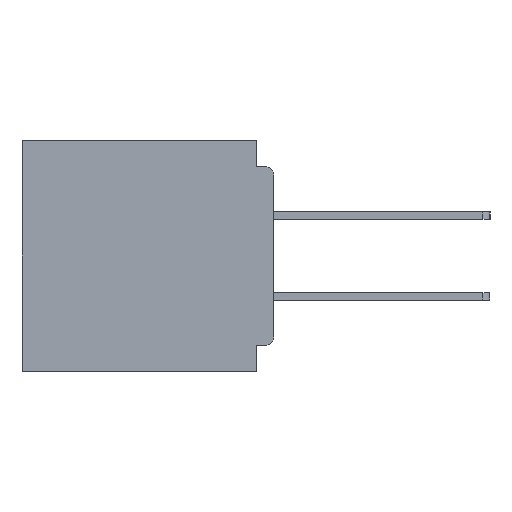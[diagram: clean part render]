
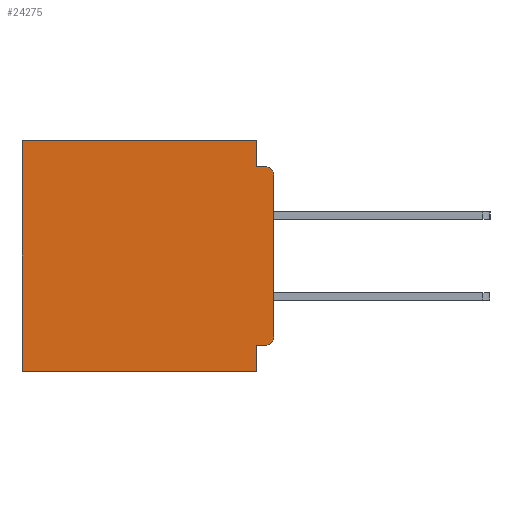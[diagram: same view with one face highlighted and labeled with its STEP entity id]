
A CAD part, left-side view. The second image highlights one B-rep face of the part: STEP entity #24275.
In plain terms, the highlighted planar face has unit normal (-1, 0, 0).
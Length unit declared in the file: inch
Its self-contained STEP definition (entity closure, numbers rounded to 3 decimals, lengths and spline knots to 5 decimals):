
#1259 = ORIENTED_EDGE ( 'NONE', *, *, #41364, .T. ) ;
#1896 = DIRECTION ( 'NONE',  ( 0., 0., -1. ) ) ;
#2210 = VECTOR ( 'NONE', #35630, 39.37008 ) ;
#3165 = CARTESIAN_POINT ( 'NONE',  ( 0.3, 0.015, -0.355 ) ) ;
#3655 = VERTEX_POINT ( 'NONE', #24168 ) ;
#3682 = AXIS2_PLACEMENT_3D ( 'NONE', #24047, #39330, #16484 ) ;
#4925 = CIRCLE ( 'NONE', #34473, 0.015 ) ;
#5330 = VERTEX_POINT ( 'NONE', #31087 ) ;
#6801 = EDGE_CURVE ( 'NONE', #7908, #34085, #31886, .T. ) ;
#6877 = LINE ( 'NONE', #7800, #17104 ) ;
#7800 = CARTESIAN_POINT ( 'NONE',  ( 0.3, 0., -0.355 ) ) ;
#7908 = VERTEX_POINT ( 'NONE', #9162 ) ;
#8068 = CARTESIAN_POINT ( 'NONE',  ( 0.3, 0., -0.4 ) ) ;
#8554 = ORIENTED_EDGE ( 'NONE', *, *, #32010, .F. ) ;
#9162 = CARTESIAN_POINT ( 'NONE',  ( 0.3, 0., -0.06 ) ) ;
#9656 = ORIENTED_EDGE ( 'NONE', *, *, #16237, .T. ) ;
#10289 = LINE ( 'NONE', #47189, #38359 ) ;
#10371 = CARTESIAN_POINT ( 'NONE',  ( 0.3, 0.015, -0.06 ) ) ;
#11651 = ORIENTED_EDGE ( 'NONE', *, *, #28597, .F. ) ;
#11797 = CARTESIAN_POINT ( 'NONE',  ( 0.3, 0., 0. ) ) ;
#12726 = CARTESIAN_POINT ( 'NONE',  ( 0.3, 0.437, -0.4 ) ) ;
#12987 = VECTOR ( 'NONE', #1896, 39.37008 ) ;
#13137 = EDGE_CURVE ( 'NONE', #5330, #17676, #21527, .T. ) ;
#14211 = DIRECTION ( 'NONE',  ( 0., 0., -1. ) ) ;
#16237 = EDGE_CURVE ( 'NONE', #43691, #34085, #44490, .T. ) ;
#16484 = DIRECTION ( 'NONE',  ( 0., 0., -1. ) ) ;
#17104 = VECTOR ( 'NONE', #34557, 39.37008 ) ;
#17636 = VERTEX_POINT ( 'NONE', #40933 ) ;
#17676 = VERTEX_POINT ( 'NONE', #19106 ) ;
#19106 = CARTESIAN_POINT ( 'NONE',  ( 0.3, 0.031, -0.4 ) ) ;
#20347 = VECTOR ( 'NONE', #34701, 39.37008 ) ;
#20806 = ORIENTED_EDGE ( 'NONE', *, *, #13137, .F. ) ;
#21331 = CARTESIAN_POINT ( 'NONE',  ( 0.3, 0., -0.34 ) ) ;
#21527 = LINE ( 'NONE', #24442, #41775 ) ;
#21607 = CARTESIAN_POINT ( 'NONE',  ( 0.3, 0.015, -0.34 ) ) ;
#24047 = CARTESIAN_POINT ( 'NONE',  ( 0.3, 0., -0.4 ) ) ;
#24168 = CARTESIAN_POINT ( 'NONE',  ( 0.3, 0.015, -0.045 ) ) ;
#24275 = ADVANCED_FACE ( 'NONE', ( #33967 ), #35515, .F. ) ;
#24442 = CARTESIAN_POINT ( 'NONE',  ( 0.3, 0.031, -0.4 ) ) ;
#25485 = DIRECTION ( 'NONE',  ( 0., 0., -1. ) ) ;
#25887 = EDGE_LOOP ( 'NONE', ( #32181, #32257, #46702, #11651, #42048, #1259, #27931, #20806, #8554, #9656 ) ) ;
#26176 = VECTOR ( 'NONE', #48220, 39.37008 ) ;
#27360 = LINE ( 'NONE', #44401, #26176 ) ;
#27374 = DIRECTION ( 'NONE',  ( 0., 0., -1. ) ) ;
#27720 = VERTEX_POINT ( 'NONE', #46425 ) ;
#27931 = ORIENTED_EDGE ( 'NONE', *, *, #38130, .F. ) ;
#28282 = DIRECTION ( 'NONE',  ( 0., 1., 0. ) ) ;
#28597 = EDGE_CURVE ( 'NONE', #27720, #44412, #33316, .T. ) ;
#29813 = EDGE_CURVE ( 'NONE', #44412, #3655, #27360, .T. ) ;
#30501 = LINE ( 'NONE', #11797, #20347 ) ;
#30678 = VERTEX_POINT ( 'NONE', #48464 ) ;
#31087 = CARTESIAN_POINT ( 'NONE',  ( 0.3, 0.031, -0.355 ) ) ;
#31886 = LINE ( 'NONE', #8068, #40784 ) ;
#32010 = EDGE_CURVE ( 'NONE', #43691, #5330, #6877, .T. ) ;
#32181 = ORIENTED_EDGE ( 'NONE', *, *, #6801, .F. ) ;
#32257 = ORIENTED_EDGE ( 'NONE', *, *, #44082, .T. ) ;
#32568 = CARTESIAN_POINT ( 'NONE',  ( 0.3, 0.031, 0. ) ) ;
#33316 = LINE ( 'NONE', #32568, #12987 ) ;
#33967 = FACE_OUTER_BOUND ( 'NONE', #25887, .T. ) ;
#34085 = VERTEX_POINT ( 'NONE', #21331 ) ;
#34473 = AXIS2_PLACEMENT_3D ( 'NONE', #10371, #37066, #14211 ) ;
#34557 = DIRECTION ( 'NONE',  ( 0., 1., 0. ) ) ;
#34701 = DIRECTION ( 'NONE',  ( 0., 1., 0. ) ) ;
#35515 = PLANE ( 'NONE',  #3682 ) ;
#35630 = DIRECTION ( 'NONE',  ( 0., 0., -1. ) ) ;
#37066 = DIRECTION ( 'NONE',  ( -1., 0., 0. ) ) ;
#38130 = EDGE_CURVE ( 'NONE', #17676, #17636, #10289, .T. ) ;
#38359 = VECTOR ( 'NONE', #28282, 39.37008 ) ;
#39330 = DIRECTION ( 'NONE',  ( 1., 0., 0. ) ) ;
#39707 = DIRECTION ( 'NONE',  ( 0., 0., -1. ) ) ;
#40552 = EDGE_CURVE ( 'NONE', #27720, #30678, #30501, .T. ) ;
#40784 = VECTOR ( 'NONE', #27374, 39.37008 ) ;
#40933 = CARTESIAN_POINT ( 'NONE',  ( 0.3, 0.437, -0.4 ) ) ;
#41364 = EDGE_CURVE ( 'NONE', #30678, #17636, #42894, .T. ) ;
#41775 = VECTOR ( 'NONE', #39707, 39.37008 ) ;
#42048 = ORIENTED_EDGE ( 'NONE', *, *, #40552, .T. ) ;
#42894 = LINE ( 'NONE', #12726, #2210 ) ;
#43691 = VERTEX_POINT ( 'NONE', #3165 ) ;
#44082 = EDGE_CURVE ( 'NONE', #7908, #3655, #4925, .T. ) ;
#44401 = CARTESIAN_POINT ( 'NONE',  ( 0.3, 0., -0.045 ) ) ;
#44412 = VERTEX_POINT ( 'NONE', #46552 ) ;
#44490 = CIRCLE ( 'NONE', #48237, 0.015 ) ;
#46425 = CARTESIAN_POINT ( 'NONE',  ( 0.3, 0.031, 0. ) ) ;
#46552 = CARTESIAN_POINT ( 'NONE',  ( 0.3, 0.031, -0.045 ) ) ;
#46702 = ORIENTED_EDGE ( 'NONE', *, *, #29813, .F. ) ;
#47189 = CARTESIAN_POINT ( 'NONE',  ( 0.3, 0., -0.4 ) ) ;
#48197 = DIRECTION ( 'NONE',  ( -1., 0., 0. ) ) ;
#48220 = DIRECTION ( 'NONE',  ( 0., -1., 0. ) ) ;
#48237 = AXIS2_PLACEMENT_3D ( 'NONE', #21607, #48197, #25485 ) ;
#48464 = CARTESIAN_POINT ( 'NONE',  ( 0.3, 0.437, 0. ) ) ;
